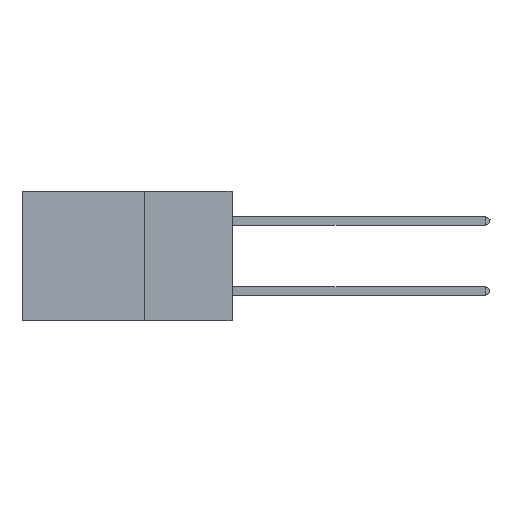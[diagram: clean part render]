
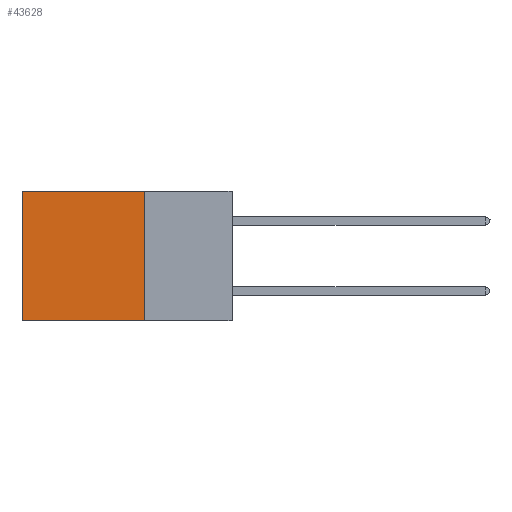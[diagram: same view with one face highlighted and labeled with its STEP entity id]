
A CAD part, left-side view. The second image highlights one B-rep face of the part: STEP entity #43628.
In plain terms, the highlighted planar face has unit normal (-1, 0, 0).
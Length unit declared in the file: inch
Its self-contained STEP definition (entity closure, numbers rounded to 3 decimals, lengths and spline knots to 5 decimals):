
#1767 = DIRECTION ( 'NONE',  ( 0., 0., -1. ) ) ;
#2861 = ORIENTED_EDGE ( 'NONE', *, *, #41540, .F. ) ;
#4515 = FACE_OUTER_BOUND ( 'NONE', #28664, .T. ) ;
#4597 = VECTOR ( 'NONE', #1767, 39.37008 ) ;
#4722 = CARTESIAN_POINT ( 'NONE',  ( 0.2875, 0.25, 0. ) ) ;
#6633 = EDGE_CURVE ( 'NONE', #23975, #7645, #16953, .T. ) ;
#6793 = CARTESIAN_POINT ( 'NONE',  ( 0.2875, 0.6, 0. ) ) ;
#7146 = DIRECTION ( 'NONE',  ( 0., 1., 0. ) ) ;
#7576 = ORIENTED_EDGE ( 'NONE', *, *, #34416, .T. ) ;
#7624 = DIRECTION ( 'NONE',  ( 0., 0., -1. ) ) ;
#7645 = VERTEX_POINT ( 'NONE', #46428 ) ;
#8276 = LINE ( 'NONE', #4722, #21477 ) ;
#10174 = DIRECTION ( 'NONE',  ( 0., 1., 0. ) ) ;
#13488 = CARTESIAN_POINT ( 'NONE',  ( 0.2875, 0.25, 0. ) ) ;
#14758 = PLANE ( 'NONE',  #23148 ) ;
#16953 = LINE ( 'NONE', #31427, #4597 ) ;
#17351 = CARTESIAN_POINT ( 'NONE',  ( 0.2875, 0.25, -0.37 ) ) ;
#17742 = ORIENTED_EDGE ( 'NONE', *, *, #20212, .F. ) ;
#19564 = ORIENTED_EDGE ( 'NONE', *, *, #6633, .T. ) ;
#20212 = EDGE_CURVE ( 'NONE', #21945, #7645, #46080, .T. ) ;
#20214 = CARTESIAN_POINT ( 'NONE',  ( 0.2875, 0.25, 0. ) ) ;
#20591 = VECTOR ( 'NONE', #7146, 39.37008 ) ;
#21281 = LINE ( 'NONE', #13488, #25919 ) ;
#21477 = VECTOR ( 'NONE', #33918, 39.37008 ) ;
#21945 = VERTEX_POINT ( 'NONE', #38204 ) ;
#22092 = DIRECTION ( 'NONE',  ( 1., 0., 0. ) ) ;
#23148 = AXIS2_PLACEMENT_3D ( 'NONE', #25647, #22092, #7624 ) ;
#23975 = VERTEX_POINT ( 'NONE', #6793 ) ;
#25647 = CARTESIAN_POINT ( 'NONE',  ( 0.2875, 0.25, 0. ) ) ;
#25919 = VECTOR ( 'NONE', #10174, 39.37008 ) ;
#28664 = EDGE_LOOP ( 'NONE', ( #19564, #17742, #2861, #7576 ) ) ;
#31427 = CARTESIAN_POINT ( 'NONE',  ( 0.2875, 0.6, 0. ) ) ;
#33918 = DIRECTION ( 'NONE',  ( 0., 0., -1. ) ) ;
#34416 = EDGE_CURVE ( 'NONE', #37090, #23975, #21281, .T. ) ;
#37090 = VERTEX_POINT ( 'NONE', #20214 ) ;
#38204 = CARTESIAN_POINT ( 'NONE',  ( 0.2875, 0.25, -0.37 ) ) ;
#41540 = EDGE_CURVE ( 'NONE', #37090, #21945, #8276, .T. ) ;
#43628 = ADVANCED_FACE ( 'NONE', ( #4515 ), #14758, .F. ) ;
#46080 = LINE ( 'NONE', #17351, #20591 ) ;
#46428 = CARTESIAN_POINT ( 'NONE',  ( 0.2875, 0.6, -0.37 ) ) ;
